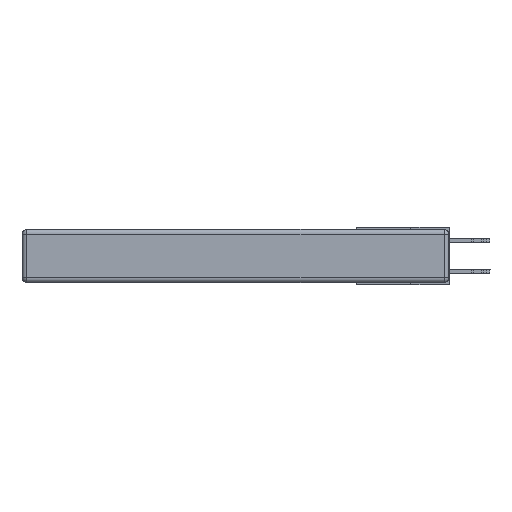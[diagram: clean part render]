
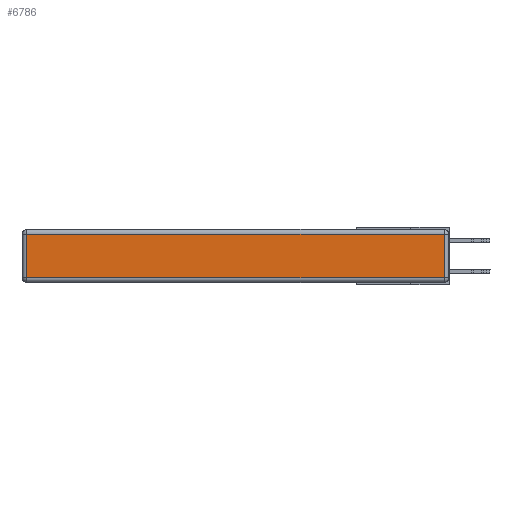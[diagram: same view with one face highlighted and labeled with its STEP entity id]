
A CAD part, left-side view. The second image highlights one B-rep face of the part: STEP entity #6786.
In plain terms, the highlighted planar face has unit normal (-1, 0, 0).
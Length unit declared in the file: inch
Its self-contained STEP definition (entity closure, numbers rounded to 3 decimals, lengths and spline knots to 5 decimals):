
#3690 = DIRECTION ( 'NONE',  ( 0., 0., -1. ) ) ;
#4171 = VECTOR ( 'NONE', #31448, 39.37008 ) ;
#4282 = VECTOR ( 'NONE', #3690, 39.37008 ) ;
#5324 = DIRECTION ( 'NONE',  ( -1., 0., 0. ) ) ;
#5488 = VECTOR ( 'NONE', #27273, 39.37008 ) ;
#5914 = VERTEX_POINT ( 'NONE', #31182 ) ;
#6378 = EDGE_LOOP ( 'NONE', ( #10143, #21051, #10552, #9770 ) ) ;
#6786 = ADVANCED_FACE ( 'NONE', ( #17209 ), #12822, .T. ) ;
#8605 = LINE ( 'NONE', #24790, #5488 ) ;
#9425 = CARTESIAN_POINT ( 'NONE',  ( 0., 2.75, -0.03 ) ) ;
#9534 = AXIS2_PLACEMENT_3D ( 'NONE', #19828, #5324, #22458 ) ;
#9770 = ORIENTED_EDGE ( 'NONE', *, *, #25069, .T. ) ;
#10143 = ORIENTED_EDGE ( 'NONE', *, *, #31377, .T. ) ;
#10552 = ORIENTED_EDGE ( 'NONE', *, *, #26424, .T. ) ;
#10917 = DIRECTION ( 'NONE',  ( 0., -1., 0. ) ) ;
#12250 = CARTESIAN_POINT ( 'NONE',  ( 0., 0., -0.313 ) ) ;
#12464 = VERTEX_POINT ( 'NONE', #29515 ) ;
#12822 = PLANE ( 'NONE',  #9534 ) ;
#15550 = LINE ( 'NONE', #28540, #4282 ) ;
#16457 = EDGE_CURVE ( 'NONE', #5914, #20906, #8605, .T. ) ;
#17209 = FACE_OUTER_BOUND ( 'NONE', #6378, .T. ) ;
#19828 = CARTESIAN_POINT ( 'NONE',  ( 0., 0., -0.343 ) ) ;
#20819 = LINE ( 'NONE', #9425, #4171 ) ;
#20906 = VERTEX_POINT ( 'NONE', #21775 ) ;
#21051 = ORIENTED_EDGE ( 'NONE', *, *, #16457, .T. ) ;
#21775 = CARTESIAN_POINT ( 'NONE',  ( 0., 0.03, -0.03 ) ) ;
#22458 = DIRECTION ( 'NONE',  ( 0., 0., 1. ) ) ;
#22491 = CARTESIAN_POINT ( 'NONE',  ( 0., 2.72, -0.313 ) ) ;
#24790 = CARTESIAN_POINT ( 'NONE',  ( 0., 0.03, -0.343 ) ) ;
#25069 = EDGE_CURVE ( 'NONE', #12464, #29122, #15550, .T. ) ;
#25572 = VECTOR ( 'NONE', #10917, 39.37008 ) ;
#26424 = EDGE_CURVE ( 'NONE', #20906, #12464, #20819, .T. ) ;
#27273 = DIRECTION ( 'NONE',  ( 0., 0., 1. ) ) ;
#27876 = LINE ( 'NONE', #12250, #25572 ) ;
#28540 = CARTESIAN_POINT ( 'NONE',  ( 0., 2.72, -0.343 ) ) ;
#29122 = VERTEX_POINT ( 'NONE', #22491 ) ;
#29515 = CARTESIAN_POINT ( 'NONE',  ( 0., 2.72, -0.03 ) ) ;
#31182 = CARTESIAN_POINT ( 'NONE',  ( 0., 0.03, -0.313 ) ) ;
#31377 = EDGE_CURVE ( 'NONE', #29122, #5914, #27876, .T. ) ;
#31448 = DIRECTION ( 'NONE',  ( 0., 1., 0. ) ) ;
